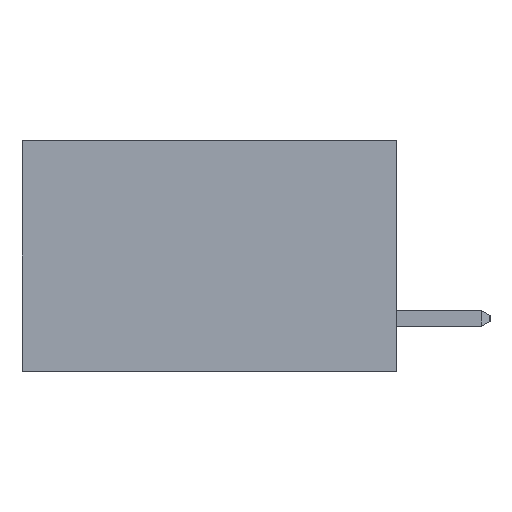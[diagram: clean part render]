
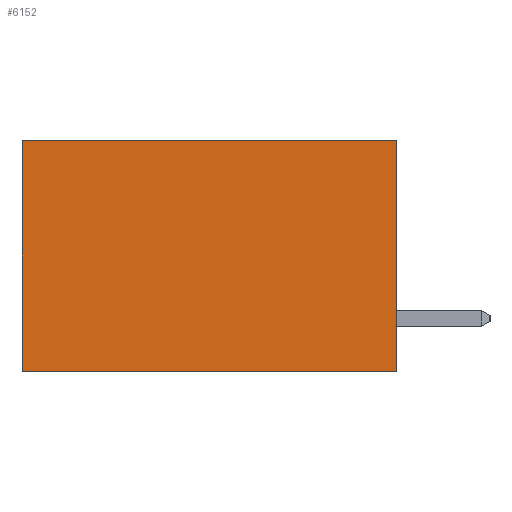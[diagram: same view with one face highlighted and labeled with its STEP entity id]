
A CAD part, left-side view. The second image highlights one B-rep face of the part: STEP entity #6152.
In plain terms, the highlighted planar face has unit normal (-1, 0, 0).
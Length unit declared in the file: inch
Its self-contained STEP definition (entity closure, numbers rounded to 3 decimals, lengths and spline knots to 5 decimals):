
#178 = PLANE ( 'NONE',  #4340 ) ;
#717 = LINE ( 'NONE', #11823, #7289 ) ;
#819 = LINE ( 'NONE', #6592, #7406 ) ;
#1194 = ORIENTED_EDGE ( 'NONE', *, *, #8823, .T. ) ;
#1396 = VERTEX_POINT ( 'NONE', #10162 ) ;
#3117 = EDGE_CURVE ( 'NONE', #10466, #4147, #3603, .T. ) ;
#3203 = EDGE_LOOP ( 'NONE', ( #1194, #6589, #14705, #14481 ) ) ;
#3603 = LINE ( 'NONE', #12852, #6660 ) ;
#4014 = DIRECTION ( 'NONE',  ( 1., 0., 0. ) ) ;
#4064 = CARTESIAN_POINT ( 'NONE',  ( 0.298, 0., -0.37 ) ) ;
#4129 = CARTESIAN_POINT ( 'NONE',  ( 0.298, 0., 0. ) ) ;
#4147 = VERTEX_POINT ( 'NONE', #5346 ) ;
#4340 = AXIS2_PLACEMENT_3D ( 'NONE', #4129, #4014, #15252 ) ;
#4843 = EDGE_CURVE ( 'NONE', #10466, #10656, #7827, .T. ) ;
#5192 = EDGE_CURVE ( 'NONE', #10656, #1396, #819, .T. ) ;
#5346 = CARTESIAN_POINT ( 'NONE',  ( 0.298, 0.6, 0. ) ) ;
#6152 = ADVANCED_FACE ( 'NONE', ( #12620 ), #178, .F. ) ;
#6589 = ORIENTED_EDGE ( 'NONE', *, *, #5192, .F. ) ;
#6592 = CARTESIAN_POINT ( 'NONE',  ( 0.298, 0., -0.37 ) ) ;
#6660 = VECTOR ( 'NONE', #13225, 39.37008 ) ;
#7289 = VECTOR ( 'NONE', #11726, 39.37008 ) ;
#7406 = VECTOR ( 'NONE', #7453, 39.37008 ) ;
#7453 = DIRECTION ( 'NONE',  ( 0., 1., 0. ) ) ;
#7827 = LINE ( 'NONE', #9004, #10064 ) ;
#8756 = CARTESIAN_POINT ( 'NONE',  ( 0.298, 0., 0. ) ) ;
#8823 = EDGE_CURVE ( 'NONE', #4147, #1396, #717, .T. ) ;
#9004 = CARTESIAN_POINT ( 'NONE',  ( 0.298, 0., 0. ) ) ;
#10064 = VECTOR ( 'NONE', #13060, 39.37008 ) ;
#10162 = CARTESIAN_POINT ( 'NONE',  ( 0.298, 0.6, -0.37 ) ) ;
#10466 = VERTEX_POINT ( 'NONE', #8756 ) ;
#10656 = VERTEX_POINT ( 'NONE', #4064 ) ;
#11726 = DIRECTION ( 'NONE',  ( 0., 0., -1. ) ) ;
#11823 = CARTESIAN_POINT ( 'NONE',  ( 0.298, 0.6, 0. ) ) ;
#12620 = FACE_OUTER_BOUND ( 'NONE', #3203, .T. ) ;
#12852 = CARTESIAN_POINT ( 'NONE',  ( 0.298, 0., 0. ) ) ;
#13060 = DIRECTION ( 'NONE',  ( 0., 0., -1. ) ) ;
#13225 = DIRECTION ( 'NONE',  ( 0., 1., 0. ) ) ;
#14481 = ORIENTED_EDGE ( 'NONE', *, *, #3117, .T. ) ;
#14705 = ORIENTED_EDGE ( 'NONE', *, *, #4843, .F. ) ;
#15252 = DIRECTION ( 'NONE',  ( 0., 0., -1. ) ) ;
